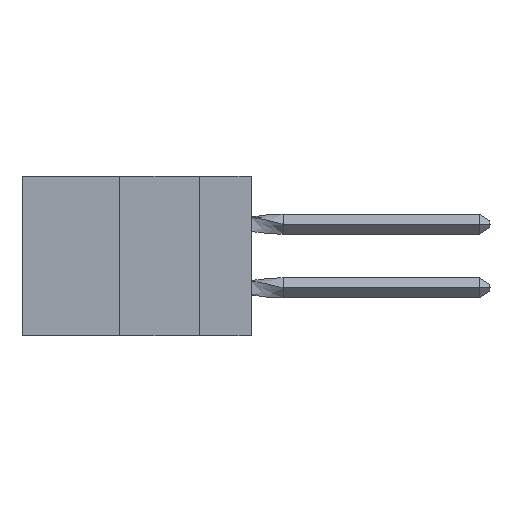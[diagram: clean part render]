
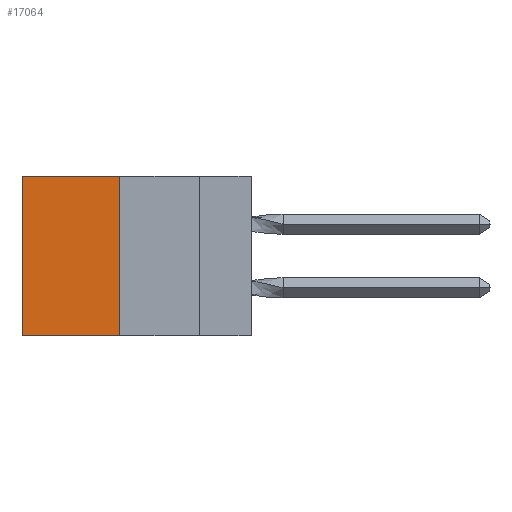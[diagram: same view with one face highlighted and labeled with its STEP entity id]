
A CAD part, left-side view. The second image highlights one B-rep face of the part: STEP entity #17064.
In plain terms, the highlighted planar face has unit normal (-1, 0, 0).
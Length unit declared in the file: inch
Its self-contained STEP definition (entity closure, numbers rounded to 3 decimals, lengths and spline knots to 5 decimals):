
#747 = CARTESIAN_POINT ( 'NONE',  ( 0.305, 0.72, -0.5 ) ) ;
#1233 = CARTESIAN_POINT ( 'NONE',  ( 0.305, 0.413, 0. ) ) ;
#2266 = DIRECTION ( 'NONE',  ( 1., 0., 0. ) ) ;
#5418 = EDGE_CURVE ( 'NONE', #17459, #33864, #6677, .T. ) ;
#6677 = LINE ( 'NONE', #15426, #24510 ) ;
#7053 = AXIS2_PLACEMENT_3D ( 'NONE', #21751, #2266, #21982 ) ;
#9416 = DIRECTION ( 'NONE',  ( 0., 1., 0. ) ) ;
#9444 = EDGE_CURVE ( 'NONE', #31481, #34717, #15082, .T. ) ;
#10415 = CARTESIAN_POINT ( 'NONE',  ( 0.305, 0.413, 0. ) ) ;
#10691 = EDGE_CURVE ( 'NONE', #33864, #34717, #33249, .T. ) ;
#12397 = ORIENTED_EDGE ( 'NONE', *, *, #9444, .T. ) ;
#15082 = LINE ( 'NONE', #25214, #33352 ) ;
#15426 = CARTESIAN_POINT ( 'NONE',  ( 0.305, 0.413, -0.5 ) ) ;
#16254 = VECTOR ( 'NONE', #22087, 39.37008 ) ;
#17064 = ADVANCED_FACE ( 'NONE', ( #27657 ), #35491, .F. ) ;
#17459 = VERTEX_POINT ( 'NONE', #10415 ) ;
#18167 = CARTESIAN_POINT ( 'NONE',  ( 0.305, 0.413, -0.5 ) ) ;
#18566 = DIRECTION ( 'NONE',  ( 0., 0., -1. ) ) ;
#19066 = CARTESIAN_POINT ( 'NONE',  ( 0.305, 0.413, -0.5 ) ) ;
#19986 = DIRECTION ( 'NONE',  ( 0., 0., -1. ) ) ;
#21751 = CARTESIAN_POINT ( 'NONE',  ( 0.305, 0.413, -0.5 ) ) ;
#21982 = DIRECTION ( 'NONE',  ( 0., 0., -1. ) ) ;
#22084 = ORIENTED_EDGE ( 'NONE', *, *, #5418, .F. ) ;
#22087 = DIRECTION ( 'NONE',  ( 0., 1., 0. ) ) ;
#23951 = LINE ( 'NONE', #1233, #35752 ) ;
#24510 = VECTOR ( 'NONE', #18566, 39.37008 ) ;
#25214 = CARTESIAN_POINT ( 'NONE',  ( 0.305, 0.72, -0.5 ) ) ;
#27657 = FACE_OUTER_BOUND ( 'NONE', #28232, .T. ) ;
#28183 = ORIENTED_EDGE ( 'NONE', *, *, #33671, .T. ) ;
#28232 = EDGE_LOOP ( 'NONE', ( #12397, #33667, #22084, #28183 ) ) ;
#31481 = VERTEX_POINT ( 'NONE', #35921 ) ;
#33249 = LINE ( 'NONE', #19066, #16254 ) ;
#33352 = VECTOR ( 'NONE', #19986, 39.37008 ) ;
#33667 = ORIENTED_EDGE ( 'NONE', *, *, #10691, .F. ) ;
#33671 = EDGE_CURVE ( 'NONE', #17459, #31481, #23951, .T. ) ;
#33864 = VERTEX_POINT ( 'NONE', #18167 ) ;
#34717 = VERTEX_POINT ( 'NONE', #747 ) ;
#35491 = PLANE ( 'NONE',  #7053 ) ;
#35752 = VECTOR ( 'NONE', #9416, 39.37008 ) ;
#35921 = CARTESIAN_POINT ( 'NONE',  ( 0.305, 0.72, 0. ) ) ;
